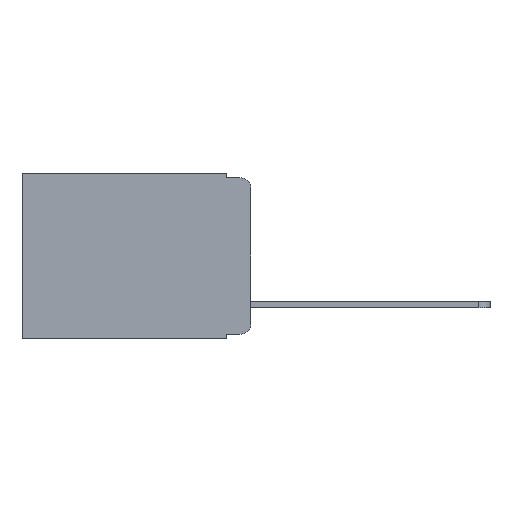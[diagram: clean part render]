
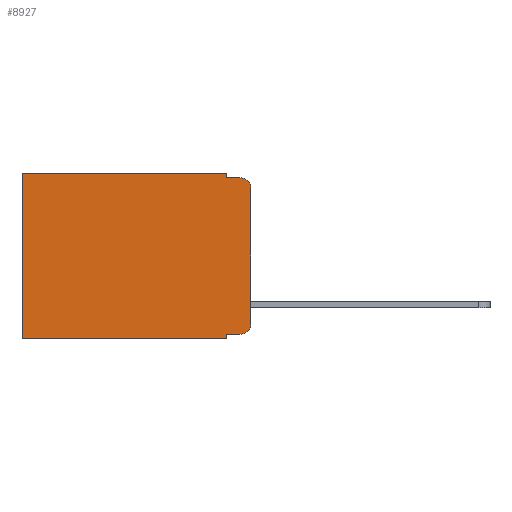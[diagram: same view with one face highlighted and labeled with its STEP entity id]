
A CAD part, left-side view. The second image highlights one B-rep face of the part: STEP entity #8927.
In plain terms, the highlighted planar face has unit normal (-1, 0, 0).
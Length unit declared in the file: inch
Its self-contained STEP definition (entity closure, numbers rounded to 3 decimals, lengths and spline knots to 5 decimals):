
#319 = CARTESIAN_POINT ( 'NONE',  ( 0.298, 0., 0. ) ) ;
#621 = ORIENTED_EDGE ( 'NONE', *, *, #23654, .T. ) ;
#740 = CARTESIAN_POINT ( 'NONE',  ( 0.298, 0., 0. ) ) ;
#1291 = DIRECTION ( 'NONE',  ( 0., 0., -1. ) ) ;
#1355 = CARTESIAN_POINT ( 'NONE',  ( 0.298, 0.02, -0.03 ) ) ;
#1871 = AXIS2_PLACEMENT_3D ( 'NONE', #5527, #21294, #19404 ) ;
#2554 = CARTESIAN_POINT ( 'NONE',  ( 0.298, 0.051, -0.333 ) ) ;
#2566 = LINE ( 'NONE', #319, #3792 ) ;
#2714 = EDGE_CURVE ( 'NONE', #12006, #11770, #22549, .T. ) ;
#2878 = LINE ( 'NONE', #2554, #24997 ) ;
#3426 = CARTESIAN_POINT ( 'NONE',  ( 0.298, 0.051, -0.343 ) ) ;
#3792 = VECTOR ( 'NONE', #21793, 39.37008 ) ;
#4062 = ORIENTED_EDGE ( 'NONE', *, *, #9996, .F. ) ;
#4229 = CARTESIAN_POINT ( 'NONE',  ( 0.298, 0.473, -0.343 ) ) ;
#4337 = LINE ( 'NONE', #8467, #10175 ) ;
#4902 = VECTOR ( 'NONE', #20080, 39.37008 ) ;
#5527 = CARTESIAN_POINT ( 'NONE',  ( 0.298, 0.02, -0.313 ) ) ;
#5721 = VERTEX_POINT ( 'NONE', #3426 ) ;
#5913 = FACE_OUTER_BOUND ( 'NONE', #20552, .T. ) ;
#5938 = ORIENTED_EDGE ( 'NONE', *, *, #6892, .T. ) ;
#6098 = ORIENTED_EDGE ( 'NONE', *, *, #19341, .F. ) ;
#6160 = LINE ( 'NONE', #740, #19942 ) ;
#6892 = EDGE_CURVE ( 'NONE', #18040, #17660, #11830, .T. ) ;
#6911 = VECTOR ( 'NONE', #24961, 39.37008 ) ;
#7166 = EDGE_CURVE ( 'NONE', #12006, #23740, #6160, .T. ) ;
#7392 = CARTESIAN_POINT ( 'NONE',  ( 0.298, 0., 0. ) ) ;
#8181 = CARTESIAN_POINT ( 'NONE',  ( 0.298, 0.051, 0. ) ) ;
#8203 = EDGE_CURVE ( 'NONE', #9265, #17660, #2566, .T. ) ;
#8467 = CARTESIAN_POINT ( 'NONE',  ( 0.298, 0.051, -0.01 ) ) ;
#8841 = CIRCLE ( 'NONE', #25411, 0.02 ) ;
#8927 = ADVANCED_FACE ( 'NONE', ( #5913 ), #24608, .F. ) ;
#9018 = ORIENTED_EDGE ( 'NONE', *, *, #9444, .F. ) ;
#9265 = VERTEX_POINT ( 'NONE', #20381 ) ;
#9444 = EDGE_CURVE ( 'NONE', #11770, #21966, #4337, .T. ) ;
#9521 = LINE ( 'NONE', #10555, #4902 ) ;
#9911 = ORIENTED_EDGE ( 'NONE', *, *, #18413, .T. ) ;
#9996 = EDGE_CURVE ( 'NONE', #5721, #15201, #10451, .T. ) ;
#10175 = VECTOR ( 'NONE', #23986, 39.37008 ) ;
#10446 = DIRECTION ( 'NONE',  ( 0., -1., 0. ) ) ;
#10451 = LINE ( 'NONE', #15965, #21527 ) ;
#10555 = CARTESIAN_POINT ( 'NONE',  ( 0.298, 0.473, 0. ) ) ;
#11518 = DIRECTION ( 'NONE',  ( 0., 0., -1. ) ) ;
#11770 = VERTEX_POINT ( 'NONE', #14006 ) ;
#11793 = VERTEX_POINT ( 'NONE', #18567 ) ;
#11830 = CIRCLE ( 'NONE', #1871, 0.02 ) ;
#12006 = VERTEX_POINT ( 'NONE', #8181 ) ;
#12644 = ORIENTED_EDGE ( 'NONE', *, *, #8203, .F. ) ;
#14006 = CARTESIAN_POINT ( 'NONE',  ( 0.298, 0.051, -0.01 ) ) ;
#14049 = CARTESIAN_POINT ( 'NONE',  ( 0.298, 0.473, 0. ) ) ;
#14341 = AXIS2_PLACEMENT_3D ( 'NONE', #7392, #20842, #1291 ) ;
#15201 = VERTEX_POINT ( 'NONE', #4229 ) ;
#15965 = CARTESIAN_POINT ( 'NONE',  ( 0.298, 0., -0.343 ) ) ;
#16532 = LINE ( 'NONE', #22685, #25424 ) ;
#17469 = CARTESIAN_POINT ( 'NONE',  ( 0.298, 0.02, -0.01 ) ) ;
#17486 = CARTESIAN_POINT ( 'NONE',  ( 0.298, 0.02, -0.333 ) ) ;
#17660 = VERTEX_POINT ( 'NONE', #22042 ) ;
#17977 = ORIENTED_EDGE ( 'NONE', *, *, #7166, .T. ) ;
#18002 = ORIENTED_EDGE ( 'NONE', *, *, #21769, .T. ) ;
#18040 = VERTEX_POINT ( 'NONE', #17486 ) ;
#18413 = EDGE_CURVE ( 'NONE', #23740, #15201, #9521, .T. ) ;
#18567 = CARTESIAN_POINT ( 'NONE',  ( 0.298, 0.051, -0.333 ) ) ;
#19341 = EDGE_CURVE ( 'NONE', #11793, #5721, #16532, .T. ) ;
#19404 = DIRECTION ( 'NONE',  ( 0., 0., -1. ) ) ;
#19942 = VECTOR ( 'NONE', #22352, 39.37008 ) ;
#20080 = DIRECTION ( 'NONE',  ( 0., 0., -1. ) ) ;
#20381 = CARTESIAN_POINT ( 'NONE',  ( 0.298, 0., -0.03 ) ) ;
#20552 = EDGE_LOOP ( 'NONE', ( #12644, #18002, #9018, #24921, #17977, #9911, #4062, #6098, #621, #5938 ) ) ;
#20842 = DIRECTION ( 'NONE',  ( 1., 0., 0. ) ) ;
#21014 = CARTESIAN_POINT ( 'NONE',  ( 0.298, 0.051, 0. ) ) ;
#21159 = DIRECTION ( 'NONE',  ( -1., 0., 0. ) ) ;
#21294 = DIRECTION ( 'NONE',  ( -1., 0., 0. ) ) ;
#21527 = VECTOR ( 'NONE', #23845, 39.37008 ) ;
#21769 = EDGE_CURVE ( 'NONE', #9265, #21966, #8841, .T. ) ;
#21793 = DIRECTION ( 'NONE',  ( 0., 0., -1. ) ) ;
#21875 = DIRECTION ( 'NONE',  ( 0., 0., -1. ) ) ;
#21966 = VERTEX_POINT ( 'NONE', #17469 ) ;
#22042 = CARTESIAN_POINT ( 'NONE',  ( 0.298, 0., -0.313 ) ) ;
#22352 = DIRECTION ( 'NONE',  ( 0., 1., 0. ) ) ;
#22549 = LINE ( 'NONE', #21014, #6911 ) ;
#22685 = CARTESIAN_POINT ( 'NONE',  ( 0.298, 0.051, 0. ) ) ;
#23654 = EDGE_CURVE ( 'NONE', #11793, #18040, #2878, .T. ) ;
#23740 = VERTEX_POINT ( 'NONE', #14049 ) ;
#23845 = DIRECTION ( 'NONE',  ( 0., 1., 0. ) ) ;
#23986 = DIRECTION ( 'NONE',  ( 0., -1., 0. ) ) ;
#24608 = PLANE ( 'NONE',  #14341 ) ;
#24921 = ORIENTED_EDGE ( 'NONE', *, *, #2714, .F. ) ;
#24961 = DIRECTION ( 'NONE',  ( 0., 0., -1. ) ) ;
#24997 = VECTOR ( 'NONE', #10446, 39.37008 ) ;
#25411 = AXIS2_PLACEMENT_3D ( 'NONE', #1355, #21159, #11518 ) ;
#25424 = VECTOR ( 'NONE', #21875, 39.37008 ) ;
